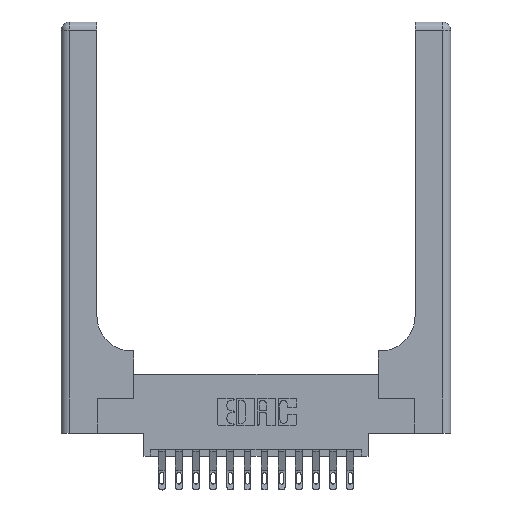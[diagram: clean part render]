
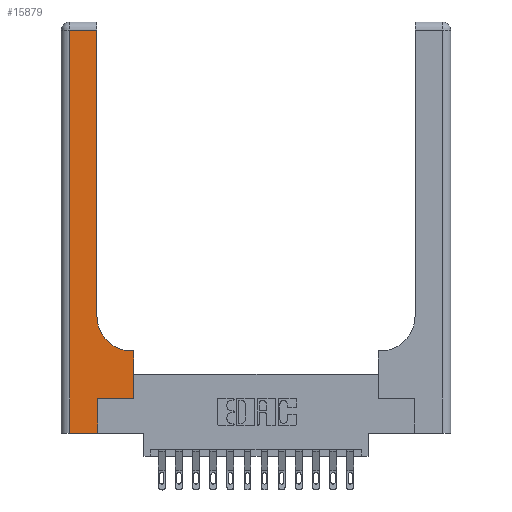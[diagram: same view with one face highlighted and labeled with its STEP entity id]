
A CAD part, top view. The second image highlights one B-rep face of the part: STEP entity #15879.
In plain terms, the highlighted planar face has unit normal (0, 0, 1).
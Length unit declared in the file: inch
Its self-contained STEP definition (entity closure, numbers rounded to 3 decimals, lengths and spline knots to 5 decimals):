
#163 = CARTESIAN_POINT ( 'NONE',  ( 0.51, 0.6, 0.37 ) ) ;
#344 = LINE ( 'NONE', #14762, #3938 ) ;
#349 = VECTOR ( 'NONE', #4054, 39.37008 ) ;
#588 = DIRECTION ( 'NONE',  ( 0., 0., -1. ) ) ;
#714 = VECTOR ( 'NONE', #3374, 39.37008 ) ;
#1614 = LINE ( 'NONE', #2682, #349 ) ;
#1671 = EDGE_CURVE ( 'NONE', #2717, #12014, #10252, .T. ) ;
#2100 = VECTOR ( 'NONE', #8700, 39.37008 ) ;
#2320 = VERTEX_POINT ( 'NONE', #5951 ) ;
#2590 = CARTESIAN_POINT ( 'NONE',  ( 0.26, 0.85, 0.37 ) ) ;
#2682 = CARTESIAN_POINT ( 'NONE',  ( 0.265, 0., 0.37 ) ) ;
#2691 = LINE ( 'NONE', #4201, #16694 ) ;
#2717 = VERTEX_POINT ( 'NONE', #12344 ) ;
#2722 = CARTESIAN_POINT ( 'NONE',  ( 0.51, 0.85, 0.37 ) ) ;
#2956 = ORIENTED_EDGE ( 'NONE', *, *, #4343, .T. ) ;
#3374 = DIRECTION ( 'NONE',  ( 1., 0., 0. ) ) ;
#3467 = VECTOR ( 'NONE', #14389, 39.37008 ) ;
#3640 = ORIENTED_EDGE ( 'NONE', *, *, #9120, .T. ) ;
#3938 = VECTOR ( 'NONE', #6673, 39.37008 ) ;
#4054 = DIRECTION ( 'NONE',  ( 0., 1., 0. ) ) ;
#4109 = DIRECTION ( 'NONE',  ( 1., 0., 0. ) ) ;
#4201 = CARTESIAN_POINT ( 'NONE',  ( 0.26, 3., 0.37 ) ) ;
#4343 = EDGE_CURVE ( 'NONE', #2320, #13200, #15137, .T. ) ;
#4460 = EDGE_CURVE ( 'NONE', #11848, #11417, #9866, .T. ) ;
#4693 = VECTOR ( 'NONE', #9317, 39.37008 ) ;
#5119 = LINE ( 'NONE', #10674, #4693 ) ;
#5627 = CARTESIAN_POINT ( 'NONE',  ( 0.06, 3., 0.37 ) ) ;
#5951 = CARTESIAN_POINT ( 'NONE',  ( 0.265, 0.25, 0.37 ) ) ;
#6146 = LINE ( 'NONE', #16792, #2100 ) ;
#6363 = ORIENTED_EDGE ( 'NONE', *, *, #9961, .T. ) ;
#6420 = AXIS2_PLACEMENT_3D ( 'NONE', #10048, #588, #10107 ) ;
#6500 = ORIENTED_EDGE ( 'NONE', *, *, #4460, .T. ) ;
#6673 = DIRECTION ( 'NONE',  ( 0., 1., 0. ) ) ;
#7068 = EDGE_CURVE ( 'NONE', #12014, #16909, #6146, .T. ) ;
#7662 = CARTESIAN_POINT ( 'NONE',  ( 0.26, 0.6, 0.37 ) ) ;
#8397 = ORIENTED_EDGE ( 'NONE', *, *, #7068, .T. ) ;
#8518 = CARTESIAN_POINT ( 'NONE',  ( 0.06, 0., 0.37 ) ) ;
#8670 = EDGE_LOOP ( 'NONE', ( #3640, #16528, #15260, #8397, #6363, #2956, #9330, #6500, #15778 ) ) ;
#8700 = DIRECTION ( 'NONE',  ( 1., 0., 0. ) ) ;
#8741 = PLANE ( 'NONE',  #6420 ) ;
#9120 = EDGE_CURVE ( 'NONE', #17528, #12698, #2691, .T. ) ;
#9317 = DIRECTION ( 'NONE',  ( -1., 0., 0. ) ) ;
#9330 = ORIENTED_EDGE ( 'NONE', *, *, #17190, .T. ) ;
#9694 = DIRECTION ( 'NONE',  ( 0., 1., 0. ) ) ;
#9866 = LINE ( 'NONE', #7662, #3467 ) ;
#9961 = EDGE_CURVE ( 'NONE', #16909, #2320, #1614, .T. ) ;
#10048 = CARTESIAN_POINT ( 'NONE',  ( 0., 3., 0.37 ) ) ;
#10107 = DIRECTION ( 'NONE',  ( -1., 0., 0. ) ) ;
#10252 = LINE ( 'NONE', #5627, #13817 ) ;
#10515 = FACE_OUTER_BOUND ( 'NONE', #8670, .T. ) ;
#10674 = CARTESIAN_POINT ( 'NONE',  ( 0., 2.94, 0.37 ) ) ;
#11219 = EDGE_CURVE ( 'NONE', #12698, #2717, #5119, .T. ) ;
#11417 = VERTEX_POINT ( 'NONE', #163 ) ;
#11848 = VERTEX_POINT ( 'NONE', #14906 ) ;
#12014 = VERTEX_POINT ( 'NONE', #8518 ) ;
#12239 = DIRECTION ( 'NONE',  ( 0., 0., -1. ) ) ;
#12344 = CARTESIAN_POINT ( 'NONE',  ( 0.06, 2.94, 0.37 ) ) ;
#12441 = CARTESIAN_POINT ( 'NONE',  ( 0.528, 0.25, 0.37 ) ) ;
#12469 = EDGE_CURVE ( 'NONE', #11417, #17528, #12577, .T. ) ;
#12501 = AXIS2_PLACEMENT_3D ( 'NONE', #2722, #12239, #4109 ) ;
#12577 = CIRCLE ( 'NONE', #12501, 0.25 ) ;
#12698 = VERTEX_POINT ( 'NONE', #12745 ) ;
#12745 = CARTESIAN_POINT ( 'NONE',  ( 0.26, 2.94, 0.37 ) ) ;
#12863 = CARTESIAN_POINT ( 'NONE',  ( 0.265, 0.25, 0.37 ) ) ;
#13200 = VERTEX_POINT ( 'NONE', #12441 ) ;
#13817 = VECTOR ( 'NONE', #15087, 39.37008 ) ;
#14069 = CARTESIAN_POINT ( 'NONE',  ( 0.265, 0., 0.37 ) ) ;
#14389 = DIRECTION ( 'NONE',  ( -1., 0., 0. ) ) ;
#14762 = CARTESIAN_POINT ( 'NONE',  ( 0.528, 0.25, 0.37 ) ) ;
#14906 = CARTESIAN_POINT ( 'NONE',  ( 0.528, 0.6, 0.37 ) ) ;
#15087 = DIRECTION ( 'NONE',  ( 0., -1., 0. ) ) ;
#15137 = LINE ( 'NONE', #12863, #714 ) ;
#15260 = ORIENTED_EDGE ( 'NONE', *, *, #1671, .T. ) ;
#15778 = ORIENTED_EDGE ( 'NONE', *, *, #12469, .T. ) ;
#15879 = ADVANCED_FACE ( 'NONE', ( #10515 ), #8741, .F. ) ;
#16528 = ORIENTED_EDGE ( 'NONE', *, *, #11219, .T. ) ;
#16694 = VECTOR ( 'NONE', #9694, 39.37008 ) ;
#16792 = CARTESIAN_POINT ( 'NONE',  ( 0., 0., 0.37 ) ) ;
#16909 = VERTEX_POINT ( 'NONE', #14069 ) ;
#17190 = EDGE_CURVE ( 'NONE', #13200, #11848, #344, .T. ) ;
#17528 = VERTEX_POINT ( 'NONE', #2590 ) ;
